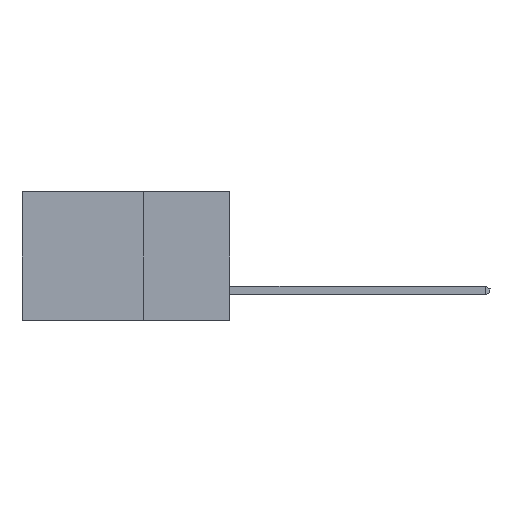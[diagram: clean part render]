
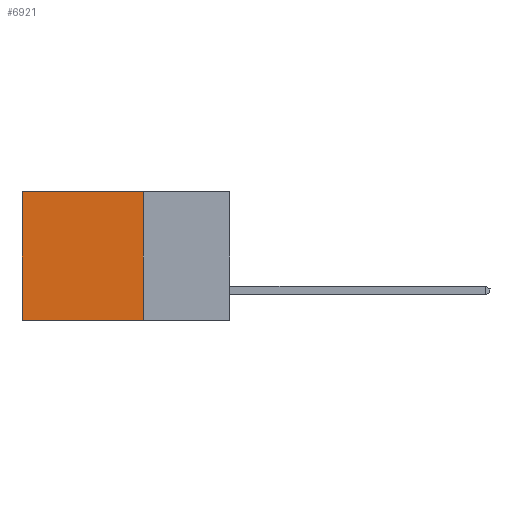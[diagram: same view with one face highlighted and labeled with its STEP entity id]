
A CAD part, left-side view. The second image highlights one B-rep face of the part: STEP entity #6921.
In plain terms, the highlighted planar face has unit normal (-1, 0, 0).
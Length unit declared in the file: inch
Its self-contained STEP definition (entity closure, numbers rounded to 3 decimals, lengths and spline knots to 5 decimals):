
#554 = DIRECTION ( 'NONE',  ( 0., 0., -1. ) ) ;
#2211 = LINE ( 'NONE', #13170, #19728 ) ;
#4604 = EDGE_CURVE ( 'NONE', #9110, #15597, #18481, .T. ) ;
#5141 = CARTESIAN_POINT ( 'NONE',  ( 0.2615, 0.6, -0.37 ) ) ;
#6045 = DIRECTION ( 'NONE',  ( 1., 0., 0. ) ) ;
#6921 = ADVANCED_FACE ( 'NONE', ( #17003 ), #17201, .F. ) ;
#7108 = LINE ( 'NONE', #7211, #18432 ) ;
#7211 = CARTESIAN_POINT ( 'NONE',  ( 0.2615, 0.6, -0.37 ) ) ;
#9110 = VERTEX_POINT ( 'NONE', #17733 ) ;
#9308 = CARTESIAN_POINT ( 'NONE',  ( 0.2615, 0.25, -0.37 ) ) ;
#10174 = DIRECTION ( 'NONE',  ( 0., 1., 0. ) ) ;
#10914 = CARTESIAN_POINT ( 'NONE',  ( 0.2615, 0.25, -0.37 ) ) ;
#11155 = ORIENTED_EDGE ( 'NONE', *, *, #4604, .F. ) ;
#11765 = VERTEX_POINT ( 'NONE', #17675 ) ;
#13170 = CARTESIAN_POINT ( 'NONE',  ( 0.2615, 0.25, -0.37 ) ) ;
#13485 = DIRECTION ( 'NONE',  ( 0., 1., 0. ) ) ;
#13621 = CARTESIAN_POINT ( 'NONE',  ( 0.2615, 0.25, -0.37 ) ) ;
#15597 = VERTEX_POINT ( 'NONE', #9308 ) ;
#15779 = VERTEX_POINT ( 'NONE', #5141 ) ;
#15811 = EDGE_CURVE ( 'NONE', #11765, #15779, #7108, .T. ) ;
#15891 = EDGE_CURVE ( 'NONE', #15597, #15779, #2211, .T. ) ;
#15904 = VECTOR ( 'NONE', #10174, 39.37008 ) ;
#16248 = CARTESIAN_POINT ( 'NONE',  ( 0.2615, 0.25, 0. ) ) ;
#16255 = AXIS2_PLACEMENT_3D ( 'NONE', #10914, #6045, #17302 ) ;
#16408 = EDGE_LOOP ( 'NONE', ( #19870, #18310, #11155, #20111 ) ) ;
#16514 = DIRECTION ( 'NONE',  ( 0., 0., -1. ) ) ;
#17003 = FACE_OUTER_BOUND ( 'NONE', #16408, .T. ) ;
#17201 = PLANE ( 'NONE',  #16255 ) ;
#17302 = DIRECTION ( 'NONE',  ( 0., 0., -1. ) ) ;
#17675 = CARTESIAN_POINT ( 'NONE',  ( 0.2615, 0.6, 0. ) ) ;
#17733 = CARTESIAN_POINT ( 'NONE',  ( 0.2615, 0.25, 0. ) ) ;
#18000 = LINE ( 'NONE', #16248, #15904 ) ;
#18310 = ORIENTED_EDGE ( 'NONE', *, *, #15891, .F. ) ;
#18432 = VECTOR ( 'NONE', #554, 39.37008 ) ;
#18481 = LINE ( 'NONE', #13621, #19785 ) ;
#19072 = EDGE_CURVE ( 'NONE', #9110, #11765, #18000, .T. ) ;
#19728 = VECTOR ( 'NONE', #13485, 39.37008 ) ;
#19785 = VECTOR ( 'NONE', #16514, 39.37008 ) ;
#19870 = ORIENTED_EDGE ( 'NONE', *, *, #15811, .T. ) ;
#20111 = ORIENTED_EDGE ( 'NONE', *, *, #19072, .T. ) ;
